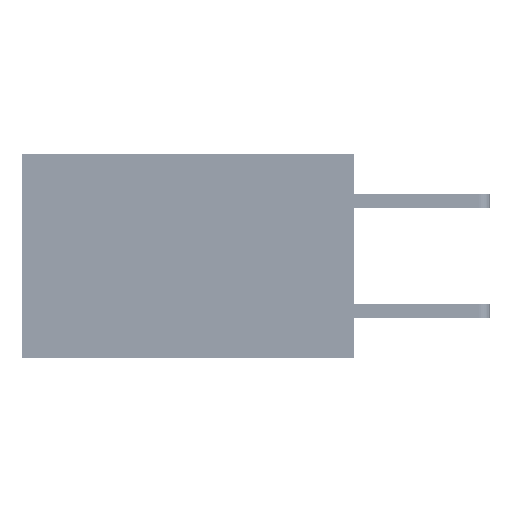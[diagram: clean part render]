
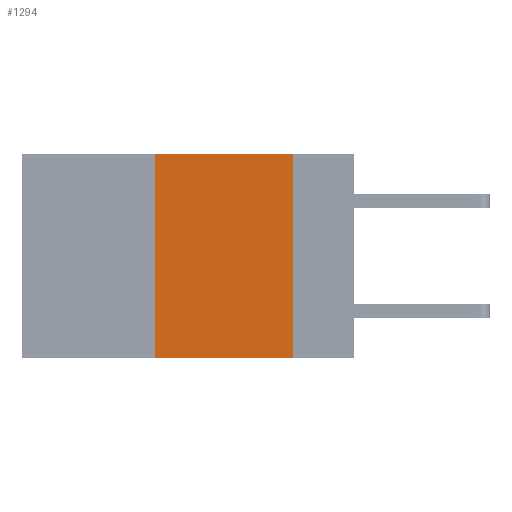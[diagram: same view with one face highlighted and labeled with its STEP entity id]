
A CAD part, left-side view. The second image highlights one B-rep face of the part: STEP entity #1294.
In plain terms, the highlighted planar face has unit normal (-1, 0, 0).
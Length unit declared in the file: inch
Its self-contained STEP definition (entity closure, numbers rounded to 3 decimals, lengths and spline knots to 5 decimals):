
#77 = VERTEX_POINT ( 'NONE', #26027 ) ;
#1294 = ADVANCED_FACE ( 'NONE', ( #18074 ), #30225, .F. ) ;
#1439 = VERTEX_POINT ( 'NONE', #41925 ) ;
#6297 = CARTESIAN_POINT ( 'NONE',  ( 0., 0.11, 0. ) ) ;
#6614 = LINE ( 'NONE', #33380, #16589 ) ;
#7874 = VECTOR ( 'NONE', #29778, 39.37008 ) ;
#8234 = VECTOR ( 'NONE', #15790, 39.37008 ) ;
#8411 = EDGE_CURVE ( 'NONE', #1439, #20849, #29215, .T. ) ;
#8714 = EDGE_CURVE ( 'NONE', #77, #18925, #6614, .T. ) ;
#8951 = EDGE_CURVE ( 'NONE', #1439, #77, #10302, .T. ) ;
#10302 = LINE ( 'NONE', #21304, #16043 ) ;
#11874 = CARTESIAN_POINT ( 'NONE',  ( 0., 0.11, -0.37 ) ) ;
#14889 = DIRECTION ( 'NONE',  ( 0., 0., 1. ) ) ;
#15790 = DIRECTION ( 'NONE',  ( 0., -1., 0. ) ) ;
#16043 = VECTOR ( 'NONE', #14889, 39.37008 ) ;
#16589 = VECTOR ( 'NONE', #16798, 39.37008 ) ;
#16798 = DIRECTION ( 'NONE',  ( 0., -1., 0. ) ) ;
#17294 = LINE ( 'NONE', #6297, #7874 ) ;
#18074 = FACE_OUTER_BOUND ( 'NONE', #31129, .T. ) ;
#18431 = AXIS2_PLACEMENT_3D ( 'NONE', #26992, #27421, #40624 ) ;
#18925 = VERTEX_POINT ( 'NONE', #20300 ) ;
#20300 = CARTESIAN_POINT ( 'NONE',  ( 0., 0.11, 0. ) ) ;
#20849 = VERTEX_POINT ( 'NONE', #11874 ) ;
#21304 = CARTESIAN_POINT ( 'NONE',  ( 0., 0.36, 0. ) ) ;
#21707 = ORIENTED_EDGE ( 'NONE', *, *, #41203, .F. ) ;
#25456 = ORIENTED_EDGE ( 'NONE', *, *, #8411, .T. ) ;
#26027 = CARTESIAN_POINT ( 'NONE',  ( 0., 0.36, 0. ) ) ;
#26992 = CARTESIAN_POINT ( 'NONE',  ( 0., 0.6, 0. ) ) ;
#27421 = DIRECTION ( 'NONE',  ( 1., 0., 0. ) ) ;
#29215 = LINE ( 'NONE', #29289, #8234 ) ;
#29289 = CARTESIAN_POINT ( 'NONE',  ( 0., 0.6, -0.37 ) ) ;
#29778 = DIRECTION ( 'NONE',  ( 0., 0., -1. ) ) ;
#29787 = ORIENTED_EDGE ( 'NONE', *, *, #8951, .F. ) ;
#30225 = PLANE ( 'NONE',  #18431 ) ;
#31129 = EDGE_LOOP ( 'NONE', ( #21707, #31680, #29787, #25456 ) ) ;
#31680 = ORIENTED_EDGE ( 'NONE', *, *, #8714, .F. ) ;
#33380 = CARTESIAN_POINT ( 'NONE',  ( 0., 0.6, 0. ) ) ;
#40624 = DIRECTION ( 'NONE',  ( 0., 0., -1. ) ) ;
#41203 = EDGE_CURVE ( 'NONE', #18925, #20849, #17294, .T. ) ;
#41925 = CARTESIAN_POINT ( 'NONE',  ( 0., 0.36, -0.37 ) ) ;
